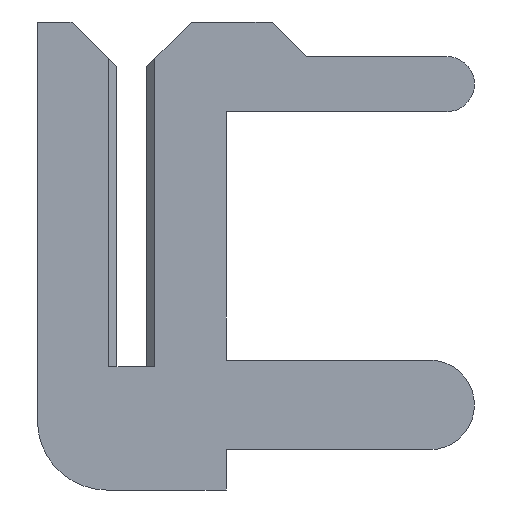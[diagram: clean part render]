
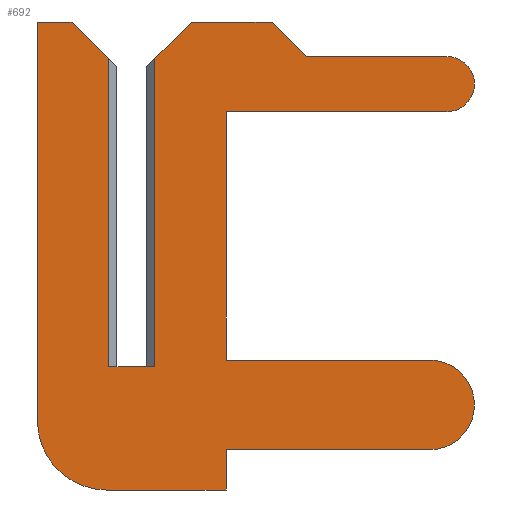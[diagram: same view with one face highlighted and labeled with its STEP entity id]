
A CAD part, left-side view. The second image highlights one B-rep face of the part: STEP entity #692.
In plain terms, the highlighted planar face has unit normal (-1, 0, 0).
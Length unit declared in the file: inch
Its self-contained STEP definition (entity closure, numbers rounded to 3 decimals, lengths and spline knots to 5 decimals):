
#8 = VECTOR ( 'NONE', #433, 39.37008 ) ;
#23 = EDGE_CURVE ( 'NONE', #469, #1033, #746, .T. ) ;
#29 = LINE ( 'NONE', #932, #8 ) ;
#39 = VERTEX_POINT ( 'NONE', #836 ) ;
#48 = VECTOR ( 'NONE', #781, 39.37008 ) ;
#53 = CARTESIAN_POINT ( 'NONE',  ( -0.01, -0.0065, 0.1305 ) ) ;
#60 = CARTESIAN_POINT ( 'NONE',  ( -0.01, 0.041, 0.15 ) ) ;
#65 = VECTOR ( 'NONE', #816, 39.37008 ) ;
#68 = VECTOR ( 'NONE', #974, 39.37008 ) ;
#74 = CARTESIAN_POINT ( 'NONE',  ( -0.01, -0.137, 0.135 ) ) ;
#75 = VERTEX_POINT ( 'NONE', #1486 ) ;
#76 = ORIENTED_EDGE ( 'NONE', *, *, #1259, .F. ) ;
#77 = EDGE_CURVE ( 'NONE', #678, #1312, #1421, .T. ) ;
#79 = DIRECTION ( 'NONE',  ( 0., -1., 0. ) ) ;
#82 = DIRECTION ( 'NONE',  ( 0., 1., 0. ) ) ;
#99 = ORIENTED_EDGE ( 'NONE', *, *, #162, .F. ) ;
#102 = VECTOR ( 'NONE', #913, 39.37008 ) ;
#118 = DIRECTION ( 'NONE',  ( 0., 0., 1. ) ) ;
#136 = VERTEX_POINT ( 'NONE', #648 ) ;
#137 = LINE ( 'NONE', #60, #65 ) ;
#162 = EDGE_CURVE ( 'NONE', #39, #178, #1135, .T. ) ;
#163 = CARTESIAN_POINT ( 'NONE',  ( -0.01, 0.011, -0.0235 ) ) ;
#178 = VERTEX_POINT ( 'NONE', #778 ) ;
#192 = ORIENTED_EDGE ( 'NONE', *, *, #1114, .F. ) ;
#197 = DIRECTION ( 'NONE',  ( 0., 0., -1. ) ) ;
#204 = CARTESIAN_POINT ( 'NONE',  ( -0.01, 0.026, 0.15 ) ) ;
#213 = ORIENTED_EDGE ( 'NONE', *, *, #896, .F. ) ;
#226 = EDGE_CURVE ( 'NONE', #791, #1195, #1525, .T. ) ;
#230 = DIRECTION ( 'NONE',  ( -1., 0., 0. ) ) ;
#251 = LINE ( 'NONE', #1304, #102 ) ;
#253 = DIRECTION ( 'NONE',  ( 0., -0.707, -0.707 ) ) ;
#256 = AXIS2_PLACEMENT_3D ( 'NONE', #1120, #355, #118 ) ;
#265 = DIRECTION ( 'NONE',  ( 0., 0., 1. ) ) ;
#270 = VERTEX_POINT ( 'NONE', #772 ) ;
#282 = ORIENTED_EDGE ( 'NONE', *, *, #1409, .F. ) ;
#290 = VECTOR ( 'NONE', #197, 39.37008 ) ;
#292 = LINE ( 'NONE', #1358, #508 ) ;
#310 = DIRECTION ( 'NONE',  ( 0., -1., 0. ) ) ;
#313 = LINE ( 'NONE', #379, #570 ) ;
#314 = DIRECTION ( 'NONE',  ( 1., 0., 0. ) ) ;
#320 = ORIENTED_EDGE ( 'NONE', *, *, #1316, .F. ) ;
#324 = CARTESIAN_POINT ( 'NONE',  ( -0.01, -0.041, 0.003 ) ) ;
#325 = CARTESIAN_POINT ( 'NONE',  ( -0.01, -0.061, 0.15 ) ) ;
#343 = LINE ( 'NONE', #1331, #631 ) ;
#345 = LINE ( 'NONE', #592, #1039 ) ;
#352 = ORIENTED_EDGE ( 'NONE', *, *, #1490, .F. ) ;
#355 = DIRECTION ( 'NONE',  ( 1., 0., 0. ) ) ;
#363 = VECTOR ( 'NONE', #310, 39.37008 ) ;
#379 = CARTESIAN_POINT ( 'NONE',  ( -0.01, -0.1295, 0.003 ) ) ;
#385 = VECTOR ( 'NONE', #265, 39.37008 ) ;
#386 = VECTOR ( 'NONE', #909, 39.37008 ) ;
#397 = ORIENTED_EDGE ( 'NONE', *, *, #1239, .F. ) ;
#403 = DIRECTION ( 'NONE',  ( 0., 0., 1. ) ) ;
#418 = LINE ( 'NONE', #1156, #48 ) ;
#425 = EDGE_CURVE ( 'NONE', #270, #469, #313, .T. ) ;
#433 = DIRECTION ( 'NONE',  ( 0., -1., 0. ) ) ;
#436 = DIRECTION ( 'NONE',  ( 0., -0.707, -0.707 ) ) ;
#447 = AXIS2_PLACEMENT_3D ( 'NONE', #1464, #230, #1308 ) ;
#451 = CARTESIAN_POINT ( 'NONE',  ( -0.01, -0.01, 0.134 ) ) ;
#463 = VECTOR ( 'NONE', #1138, 39.37008 ) ;
#469 = VERTEX_POINT ( 'NONE', #1241 ) ;
#483 = CARTESIAN_POINT ( 'NONE',  ( -0.01, 0.0065, 0.1305 ) ) ;
#508 = VECTOR ( 'NONE', #1337, 39.37008 ) ;
#537 = VERTEX_POINT ( 'NONE', #1027 ) ;
#548 = CARTESIAN_POINT ( 'NONE',  ( -0.01, -0.137, 0.111 ) ) ;
#570 = VECTOR ( 'NONE', #728, 39.37008 ) ;
#580 = CARTESIAN_POINT ( 'NONE',  ( -0.01, 0.01, 0.134 ) ) ;
#588 = ORIENTED_EDGE ( 'NONE', *, *, #1002, .F. ) ;
#592 = CARTESIAN_POINT ( 'NONE',  ( -0.01, -0.041, 0.111 ) ) ;
#600 = VERTEX_POINT ( 'NONE', #1287 ) ;
#603 = LINE ( 'NONE', #1475, #68 ) ;
#624 = EDGE_CURVE ( 'NONE', #843, #537, #1084, .T. ) ;
#631 = VECTOR ( 'NONE', #436, 39.37008 ) ;
#641 = VERTEX_POINT ( 'NONE', #1279 ) ;
#648 = CARTESIAN_POINT ( 'NONE',  ( -0.01, -0.01, 0. ) ) ;
#667 = CARTESIAN_POINT ( 'NONE',  ( -0.01, 0.0065, 0. ) ) ;
#678 = VERTEX_POINT ( 'NONE', #204 ) ;
#688 = LINE ( 'NONE', #667, #363 ) ;
#692 = ADVANCED_FACE ( 'NONE', ( #1205 ), #1336, .T. ) ;
#714 = CARTESIAN_POINT ( 'NONE',  ( -0.01, -0.1295, -0.0165 ) ) ;
#727 = AXIS2_PLACEMENT_3D ( 'NONE', #714, #314, #1219 ) ;
#728 = DIRECTION ( 'NONE',  ( 0., -1., 0. ) ) ;
#730 = ORIENTED_EDGE ( 'NONE', *, *, #1183, .F. ) ;
#746 = CIRCLE ( 'NONE', #727, 0.0195 ) ;
#761 = EDGE_CURVE ( 'NONE', #1195, #892, #345, .T. ) ;
#764 = CARTESIAN_POINT ( 'NONE',  ( -0.01, -0.041, -0.036 ) ) ;
#772 = CARTESIAN_POINT ( 'NONE',  ( -0.01, -0.041, 0.003 ) ) ;
#778 = CARTESIAN_POINT ( 'NONE',  ( -0.01, 0.041, -0.0235 ) ) ;
#781 = DIRECTION ( 'NONE',  ( 0., 1., 0. ) ) ;
#791 = VERTEX_POINT ( 'NONE', #1321 ) ;
#816 = DIRECTION ( 'NONE',  ( 0., 0., 1. ) ) ;
#820 = EDGE_CURVE ( 'NONE', #843, #136, #603, .T. ) ;
#822 = CARTESIAN_POINT ( 'NONE',  ( -0.01, -0.041, -0.0535 ) ) ;
#826 = LINE ( 'NONE', #324, #290 ) ;
#836 = CARTESIAN_POINT ( 'NONE',  ( -0.01, 0.011, -0.0535 ) ) ;
#843 = VERTEX_POINT ( 'NONE', #451 ) ;
#864 = LINE ( 'NONE', #1399, #385 ) ;
#892 = VERTEX_POINT ( 'NONE', #978 ) ;
#896 = EDGE_CURVE ( 'NONE', #75, #1412, #292, .T. ) ;
#897 = ORIENTED_EDGE ( 'NONE', *, *, #23, .F. ) ;
#909 = DIRECTION ( 'NONE',  ( 0., -0.707, 0.707 ) ) ;
#912 = AXIS2_PLACEMENT_3D ( 'NONE', #163, #1153, #403 ) ;
#913 = DIRECTION ( 'NONE',  ( 0., -1., 0. ) ) ;
#927 = CARTESIAN_POINT ( 'NONE',  ( -0.01, -0.076, 0.135 ) ) ;
#932 = CARTESIAN_POINT ( 'NONE',  ( -0.01, -0.026, 0.15 ) ) ;
#944 = ORIENTED_EDGE ( 'NONE', *, *, #226, .F. ) ;
#954 = ORIENTED_EDGE ( 'NONE', *, *, #1032, .T. ) ;
#956 = VECTOR ( 'NONE', #79, 39.37008 ) ;
#974 = DIRECTION ( 'NONE',  ( 0., 0., -1. ) ) ;
#978 = CARTESIAN_POINT ( 'NONE',  ( -0.01, -0.041, 0.111 ) ) ;
#1002 = EDGE_CURVE ( 'NONE', #1033, #75, #1016, .T. ) ;
#1012 = ORIENTED_EDGE ( 'NONE', *, *, #820, .T. ) ;
#1016 = LINE ( 'NONE', #764, #463 ) ;
#1027 = CARTESIAN_POINT ( 'NONE',  ( -0.01, -0.026, 0.15 ) ) ;
#1032 = EDGE_CURVE ( 'NONE', #600, #1312, #864, .T. ) ;
#1033 = VERTEX_POINT ( 'NONE', #1515 ) ;
#1039 = VECTOR ( 'NONE', #82, 39.37008 ) ;
#1084 = LINE ( 'NONE', #53, #386 ) ;
#1114 = EDGE_CURVE ( 'NONE', #641, #678, #251, .T. ) ;
#1120 = CARTESIAN_POINT ( 'NONE',  ( -0.01, -0.137, 0.123 ) ) ;
#1135 = CIRCLE ( 'NONE', #912, 0.03 ) ;
#1138 = DIRECTION ( 'NONE',  ( 0., 1., 0. ) ) ;
#1152 = ORIENTED_EDGE ( 'NONE', *, *, #624, .F. ) ;
#1153 = DIRECTION ( 'NONE',  ( 1., 0., 0. ) ) ;
#1156 = CARTESIAN_POINT ( 'NONE',  ( -0.01, 0.011, -0.0535 ) ) ;
#1183 = EDGE_CURVE ( 'NONE', #600, #136, #688, .T. ) ;
#1195 = VERTEX_POINT ( 'NONE', #548 ) ;
#1205 = FACE_OUTER_BOUND ( 'NONE', #1561, .T. ) ;
#1213 = ORIENTED_EDGE ( 'NONE', *, *, #1429, .F. ) ;
#1219 = DIRECTION ( 'NONE',  ( 0., 0., 1. ) ) ;
#1239 = EDGE_CURVE ( 'NONE', #1412, #39, #418, .T. ) ;
#1241 = CARTESIAN_POINT ( 'NONE',  ( -0.01, -0.1295, 0.003 ) ) ;
#1259 = EDGE_CURVE ( 'NONE', #178, #641, #137, .T. ) ;
#1279 = CARTESIAN_POINT ( 'NONE',  ( -0.01, 0.041, 0.15 ) ) ;
#1287 = CARTESIAN_POINT ( 'NONE',  ( -0.01, 0.01, 0. ) ) ;
#1302 = LINE ( 'NONE', #74, #956 ) ;
#1304 = CARTESIAN_POINT ( 'NONE',  ( -0.01, 0.026, 0.15 ) ) ;
#1308 = DIRECTION ( 'NONE',  ( 0., 0., 1. ) ) ;
#1312 = VERTEX_POINT ( 'NONE', #580 ) ;
#1316 = EDGE_CURVE ( 'NONE', #537, #1517, #29, .T. ) ;
#1317 = VECTOR ( 'NONE', #253, 39.37008 ) ;
#1321 = CARTESIAN_POINT ( 'NONE',  ( -0.01, -0.137, 0.135 ) ) ;
#1331 = CARTESIAN_POINT ( 'NONE',  ( -0.01, -0.076, 0.135 ) ) ;
#1336 = PLANE ( 'NONE',  #447 ) ;
#1337 = DIRECTION ( 'NONE',  ( 0., 0., -1. ) ) ;
#1358 = CARTESIAN_POINT ( 'NONE',  ( -0.01, -0.041, -0.0535 ) ) ;
#1369 = VERTEX_POINT ( 'NONE', #927 ) ;
#1399 = CARTESIAN_POINT ( 'NONE',  ( -0.01, 0.01, -0.0235 ) ) ;
#1409 = EDGE_CURVE ( 'NONE', #1369, #791, #1302, .T. ) ;
#1412 = VERTEX_POINT ( 'NONE', #822 ) ;
#1421 = LINE ( 'NONE', #483, #1317 ) ;
#1429 = EDGE_CURVE ( 'NONE', #1517, #1369, #343, .T. ) ;
#1433 = ORIENTED_EDGE ( 'NONE', *, *, #425, .F. ) ;
#1446 = ORIENTED_EDGE ( 'NONE', *, *, #77, .F. ) ;
#1464 = CARTESIAN_POINT ( 'NONE',  ( -0.01, 0.011, -0.0235 ) ) ;
#1475 = CARTESIAN_POINT ( 'NONE',  ( -0.01, -0.01, 0.15 ) ) ;
#1486 = CARTESIAN_POINT ( 'NONE',  ( -0.01, -0.041, -0.036 ) ) ;
#1490 = EDGE_CURVE ( 'NONE', #892, #270, #826, .T. ) ;
#1515 = CARTESIAN_POINT ( 'NONE',  ( -0.01, -0.1295, -0.036 ) ) ;
#1517 = VERTEX_POINT ( 'NONE', #325 ) ;
#1525 = CIRCLE ( 'NONE', #256, 0.012 ) ;
#1561 = EDGE_LOOP ( 'NONE', ( #1152, #1012, #730, #954, #1446, #192, #76, #99, #397, #213, #588, #897, #1433, #352, #1571, #944, #282, #1213, #320 ) ) ;
#1571 = ORIENTED_EDGE ( 'NONE', *, *, #761, .F. ) ;
